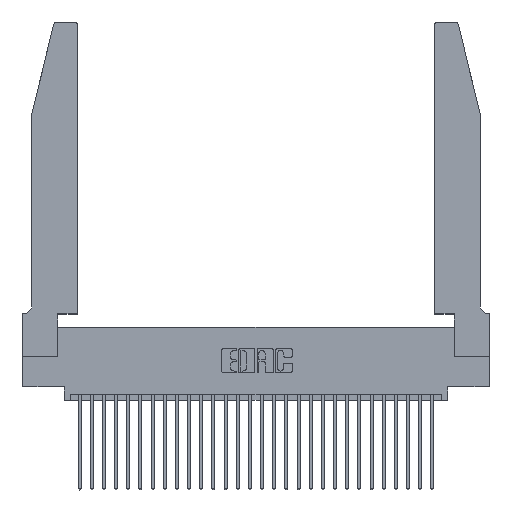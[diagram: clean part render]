
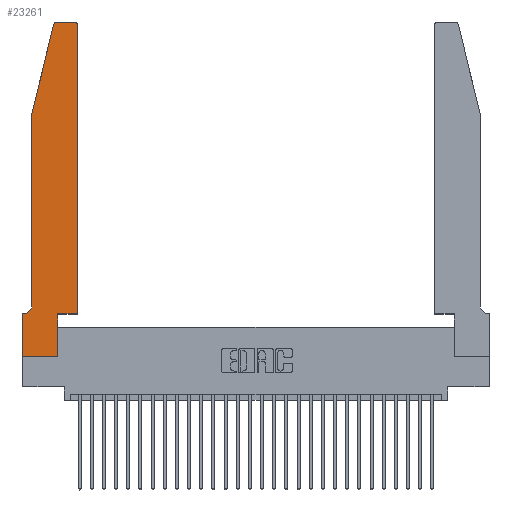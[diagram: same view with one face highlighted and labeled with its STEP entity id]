
A CAD part, top view. The second image highlights one B-rep face of the part: STEP entity #23261.
In plain terms, the highlighted planar face has unit normal (0, 0, 1).
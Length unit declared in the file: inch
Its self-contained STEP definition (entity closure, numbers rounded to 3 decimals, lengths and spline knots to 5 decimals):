
#411 = VECTOR ( 'NONE', #29353, 39.37008 ) ;
#794 = ORIENTED_EDGE ( 'NONE', *, *, #14097, .T. ) ;
#1266 = ORIENTED_EDGE ( 'NONE', *, *, #24128, .T. ) ;
#1433 = LINE ( 'NONE', #6587, #9120 ) ;
#1466 = VERTEX_POINT ( 'NONE', #15180 ) ;
#2285 = VECTOR ( 'NONE', #15941, 39.37008 ) ;
#2348 = VECTOR ( 'NONE', #22592, 39.37008 ) ;
#2486 = CIRCLE ( 'NONE', #28231, 0.03 ) ;
#2554 = CARTESIAN_POINT ( 'NONE',  ( 0.0755, 2., 0.37 ) ) ;
#2627 = LINE ( 'NONE', #18362, #2285 ) ;
#2767 = CIRCLE ( 'NONE', #3680, 0.03 ) ;
#2840 = VECTOR ( 'NONE', #13247, 39.37008 ) ;
#2972 = FACE_OUTER_BOUND ( 'NONE', #7757, .T. ) ;
#3113 = VERTEX_POINT ( 'NONE', #19312 ) ;
#3680 = AXIS2_PLACEMENT_3D ( 'NONE', #23033, #20539, #4372 ) ;
#3726 = VERTEX_POINT ( 'NONE', #4647 ) ;
#3837 = EDGE_CURVE ( 'NONE', #25365, #3113, #7024, .T. ) ;
#4257 = CIRCLE ( 'NONE', #19532, 0.07 ) ;
#4372 = DIRECTION ( 'NONE',  ( 1., 0., 0. ) ) ;
#4438 = DIRECTION ( 'NONE',  ( 0., 0., -1. ) ) ;
#4647 = CARTESIAN_POINT ( 'NONE',  ( 0.2865, 0., 0.37 ) ) ;
#4750 = CARTESIAN_POINT ( 'NONE',  ( 0.0755, 2., 0.37 ) ) ;
#5058 = DIRECTION ( 'NONE',  ( 1., 0., 0. ) ) ;
#5078 = DIRECTION ( 'NONE',  ( -0.239, -0.971, 0. ) ) ;
#5667 = EDGE_CURVE ( 'NONE', #1466, #16356, #1433, .T. ) ;
#6250 = VERTEX_POINT ( 'NONE', #15863 ) ;
#6261 = DIRECTION ( 'NONE',  ( 0., 0., 1. ) ) ;
#6546 = VECTOR ( 'NONE', #5078, 39.37008 ) ;
#6576 = DIRECTION ( 'NONE',  ( 1., 0., 0. ) ) ;
#6587 = CARTESIAN_POINT ( 'NONE',  ( 0.2605, 2.75, 0.37 ) ) ;
#6789 = CARTESIAN_POINT ( 'NONE',  ( 0.0055, 0.42, 0.37 ) ) ;
#6803 = CARTESIAN_POINT ( 'NONE',  ( 0.284, 2.75, 0.37 ) ) ;
#7003 = AXIS2_PLACEMENT_3D ( 'NONE', #22474, #6261, #6576 ) ;
#7024 = LINE ( 'NONE', #22972, #29166 ) ;
#7335 = EDGE_CURVE ( 'NONE', #17872, #17134, #20266, .T. ) ;
#7627 = CARTESIAN_POINT ( 'NONE',  ( 0.4505, 0.35, 0.37 ) ) ;
#7757 = EDGE_LOOP ( 'NONE', ( #10720, #30061, #1266, #27124, #9526, #16263, #24867, #23361, #794, #12532, #21311, #9513 ) ) ;
#8234 = CARTESIAN_POINT ( 'NONE',  ( 0.0755, 0.35, 0.37 ) ) ;
#8313 = EDGE_CURVE ( 'NONE', #16356, #16474, #2767, .T. ) ;
#9039 = CARTESIAN_POINT ( 'NONE',  ( 0., 0., 0.37 ) ) ;
#9120 = VECTOR ( 'NONE', #18501, 39.37008 ) ;
#9289 = LINE ( 'NONE', #9039, #2348 ) ;
#9513 = ORIENTED_EDGE ( 'NONE', *, *, #10875, .T. ) ;
#9526 = ORIENTED_EDGE ( 'NONE', *, *, #26840, .T. ) ;
#9585 = CARTESIAN_POINT ( 'NONE',  ( 0.4205, 2.72, 0.37 ) ) ;
#9776 = CARTESIAN_POINT ( 'NONE',  ( 0.0755, 0.42, 0.37 ) ) ;
#10434 = DIRECTION ( 'NONE',  ( 0., -1., 0. ) ) ;
#10720 = ORIENTED_EDGE ( 'NONE', *, *, #5667, .T. ) ;
#10875 = EDGE_CURVE ( 'NONE', #19016, #1466, #2486, .T. ) ;
#12134 = LINE ( 'NONE', #8234, #411 ) ;
#12344 = LINE ( 'NONE', #15483, #2840 ) ;
#12532 = ORIENTED_EDGE ( 'NONE', *, *, #3837, .T. ) ;
#12910 = CARTESIAN_POINT ( 'NONE',  ( 0.2865, 0.35, 0.37 ) ) ;
#13247 = DIRECTION ( 'NONE',  ( 0., -1., 0. ) ) ;
#14065 = CARTESIAN_POINT ( 'NONE',  ( 0., 0.35, 0.37 ) ) ;
#14097 = EDGE_CURVE ( 'NONE', #3726, #25365, #2627, .T. ) ;
#14504 = EDGE_CURVE ( 'NONE', #6250, #17888, #12134, .T. ) ;
#15180 = CARTESIAN_POINT ( 'NONE',  ( 0.4205, 2.75, 0.37 ) ) ;
#15190 = VECTOR ( 'NONE', #10434, 39.37008 ) ;
#15483 = CARTESIAN_POINT ( 'NONE',  ( 0., 0., 0.37 ) ) ;
#15540 = PLANE ( 'NONE',  #7003 ) ;
#15863 = CARTESIAN_POINT ( 'NONE',  ( 0.0055, 0.35, 0.37 ) ) ;
#15941 = DIRECTION ( 'NONE',  ( 0., 1., 0. ) ) ;
#16263 = ORIENTED_EDGE ( 'NONE', *, *, #14504, .T. ) ;
#16356 = VERTEX_POINT ( 'NONE', #6803 ) ;
#16474 = VERTEX_POINT ( 'NONE', #24189 ) ;
#16706 = EDGE_CURVE ( 'NONE', #17888, #28471, #12344, .T. ) ;
#16947 = EDGE_CURVE ( 'NONE', #3113, #19016, #25023, .T. ) ;
#17134 = VERTEX_POINT ( 'NONE', #9776 ) ;
#17872 = VERTEX_POINT ( 'NONE', #4750 ) ;
#17888 = VERTEX_POINT ( 'NONE', #14065 ) ;
#18362 = CARTESIAN_POINT ( 'NONE',  ( 0.2865, 0.35, 0.37 ) ) ;
#18501 = DIRECTION ( 'NONE',  ( -1., 0., 0. ) ) ;
#19016 = VERTEX_POINT ( 'NONE', #25283 ) ;
#19312 = CARTESIAN_POINT ( 'NONE',  ( 0.4505, 0.35, 0.37 ) ) ;
#19532 = AXIS2_PLACEMENT_3D ( 'NONE', #6789, #4438, #23012 ) ;
#20266 = LINE ( 'NONE', #24637, #15190 ) ;
#20539 = DIRECTION ( 'NONE',  ( 0., 0., 1. ) ) ;
#21311 = ORIENTED_EDGE ( 'NONE', *, *, #16947, .T. ) ;
#22205 = LINE ( 'NONE', #2554, #6546 ) ;
#22474 = CARTESIAN_POINT ( 'NONE',  ( 0., 0.35, 0.37 ) ) ;
#22592 = DIRECTION ( 'NONE',  ( 1., 0., 0. ) ) ;
#22972 = CARTESIAN_POINT ( 'NONE',  ( 0.4505, 0.35, 0.37 ) ) ;
#23012 = DIRECTION ( 'NONE',  ( -1., 0., 0. ) ) ;
#23033 = CARTESIAN_POINT ( 'NONE',  ( 0.284, 2.72, 0.37 ) ) ;
#23261 = ADVANCED_FACE ( 'NONE', ( #2972 ), #15540, .T. ) ;
#23361 = ORIENTED_EDGE ( 'NONE', *, *, #27989, .T. ) ;
#23657 = DIRECTION ( 'NONE',  ( 0., 1., 0. ) ) ;
#23721 = DIRECTION ( 'NONE',  ( 0., 0., 1. ) ) ;
#24128 = EDGE_CURVE ( 'NONE', #16474, #17872, #22205, .T. ) ;
#24189 = CARTESIAN_POINT ( 'NONE',  ( 0.25487, 2.72718, 0.37 ) ) ;
#24533 = DIRECTION ( 'NONE',  ( 1., 0., 0. ) ) ;
#24637 = CARTESIAN_POINT ( 'NONE',  ( 0.0755, 2., 0.37 ) ) ;
#24867 = ORIENTED_EDGE ( 'NONE', *, *, #16706, .T. ) ;
#25023 = LINE ( 'NONE', #7627, #26069 ) ;
#25283 = CARTESIAN_POINT ( 'NONE',  ( 0.4505, 2.72, 0.37 ) ) ;
#25365 = VERTEX_POINT ( 'NONE', #12910 ) ;
#26069 = VECTOR ( 'NONE', #23657, 39.37008 ) ;
#26840 = EDGE_CURVE ( 'NONE', #17134, #6250, #4257, .T. ) ;
#27124 = ORIENTED_EDGE ( 'NONE', *, *, #7335, .T. ) ;
#27989 = EDGE_CURVE ( 'NONE', #28471, #3726, #9289, .T. ) ;
#28231 = AXIS2_PLACEMENT_3D ( 'NONE', #9585, #23721, #5058 ) ;
#28471 = VERTEX_POINT ( 'NONE', #29261 ) ;
#29166 = VECTOR ( 'NONE', #24533, 39.37008 ) ;
#29261 = CARTESIAN_POINT ( 'NONE',  ( 0., 0., 0.37 ) ) ;
#29353 = DIRECTION ( 'NONE',  ( -1., 0., 0. ) ) ;
#30061 = ORIENTED_EDGE ( 'NONE', *, *, #8313, .T. ) ;
